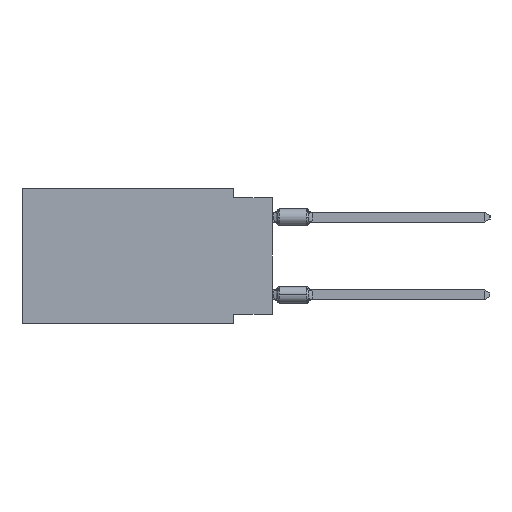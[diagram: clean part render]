
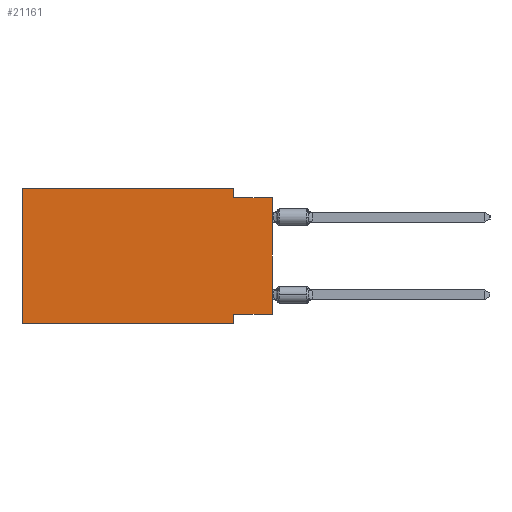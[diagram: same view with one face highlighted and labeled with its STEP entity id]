
A CAD part, left-side view. The second image highlights one B-rep face of the part: STEP entity #21161.
In plain terms, the highlighted planar face has unit normal (-1, 0, 0).
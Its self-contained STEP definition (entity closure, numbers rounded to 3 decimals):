
#135 = ORIENTED_EDGE ( 'NONE', *, *, #12241, .F. ) ;
#281 = EDGE_CURVE ( 'NONE', #18312, #9924, #28892, .T. ) ;
#1151 = CARTESIAN_POINT ( 'NONE',  ( 0., 0., -0.635 ) ) ;
#1558 = EDGE_CURVE ( 'NONE', #11872, #26297, #2142, .T. ) ;
#2047 = CARTESIAN_POINT ( 'NONE',  ( 0., 0., -8.255 ) ) ;
#2142 = LINE ( 'NONE', #33585, #17754 ) ;
#2963 = CARTESIAN_POINT ( 'NONE',  ( 0., 16.383, 0. ) ) ;
#4011 = CARTESIAN_POINT ( 'NONE',  ( 0., 16.383, -8.89 ) ) ;
#4338 = EDGE_CURVE ( 'NONE', #34104, #12734, #29491, .T. ) ;
#5373 = ORIENTED_EDGE ( 'NONE', *, *, #23506, .F. ) ;
#5751 = CARTESIAN_POINT ( 'NONE',  ( 0., 2.54, 0. ) ) ;
#7100 = EDGE_CURVE ( 'NONE', #11872, #12324, #21355, .T. ) ;
#7386 = VECTOR ( 'NONE', #18073, 1000. ) ;
#7520 = LINE ( 'NONE', #28800, #7386 ) ;
#7662 = EDGE_LOOP ( 'NONE', ( #23647, #9031, #10416, #135, #21304, #28058, #5373, #12961 ) ) ;
#8340 = DIRECTION ( 'NONE',  ( 1., 0., 0. ) ) ;
#8524 = DIRECTION ( 'NONE',  ( 0., 0., -1. ) ) ;
#8633 = EDGE_CURVE ( 'NONE', #18312, #16953, #19740, .T. ) ;
#9031 = ORIENTED_EDGE ( 'NONE', *, *, #22091, .F. ) ;
#9840 = DIRECTION ( 'NONE',  ( 0., 0., -1. ) ) ;
#9924 = VERTEX_POINT ( 'NONE', #2963 ) ;
#10416 = ORIENTED_EDGE ( 'NONE', *, *, #4338, .F. ) ;
#10452 = CARTESIAN_POINT ( 'NONE',  ( 0., 2.54, -8.89 ) ) ;
#10765 = FACE_OUTER_BOUND ( 'NONE', #7662, .T. ) ;
#11872 = VERTEX_POINT ( 'NONE', #2047 ) ;
#11925 = CARTESIAN_POINT ( 'NONE',  ( 0., 0., -0.635 ) ) ;
#12241 = EDGE_CURVE ( 'NONE', #9924, #34104, #7520, .T. ) ;
#12324 = VERTEX_POINT ( 'NONE', #13564 ) ;
#12609 = CARTESIAN_POINT ( 'NONE',  ( 0., 16.383, 0. ) ) ;
#12734 = VERTEX_POINT ( 'NONE', #18708 ) ;
#12784 = AXIS2_PLACEMENT_3D ( 'NONE', #31692, #8340, #8524 ) ;
#12961 = ORIENTED_EDGE ( 'NONE', *, *, #7100, .F. ) ;
#13564 = CARTESIAN_POINT ( 'NONE',  ( 0., 2.54, -8.255 ) ) ;
#16063 = VECTOR ( 'NONE', #9840, 1000. ) ;
#16627 = VECTOR ( 'NONE', #30184, 1000. ) ;
#16953 = VERTEX_POINT ( 'NONE', #10452 ) ;
#17480 = CARTESIAN_POINT ( 'NONE',  ( 0., 2.54, -8.89 ) ) ;
#17754 = VECTOR ( 'NONE', #28763, 1000. ) ;
#18073 = DIRECTION ( 'NONE',  ( 0., -1., 0. ) ) ;
#18312 = VERTEX_POINT ( 'NONE', #34023 ) ;
#18708 = CARTESIAN_POINT ( 'NONE',  ( 0., 2.54, -0.635 ) ) ;
#19740 = LINE ( 'NONE', #4011, #24284 ) ;
#21161 = ADVANCED_FACE ( 'NONE', ( #10765 ), #21316, .F. ) ;
#21304 = ORIENTED_EDGE ( 'NONE', *, *, #281, .F. ) ;
#21316 = PLANE ( 'NONE',  #12784 ) ;
#21355 = LINE ( 'NONE', #31887, #28816 ) ;
#22091 = EDGE_CURVE ( 'NONE', #12734, #26297, #28084, .T. ) ;
#22669 = VECTOR ( 'NONE', #23172, 1000. ) ;
#23172 = DIRECTION ( 'NONE',  ( 0., 0., 1. ) ) ;
#23506 = EDGE_CURVE ( 'NONE', #12324, #16953, #33042, .T. ) ;
#23647 = ORIENTED_EDGE ( 'NONE', *, *, #1558, .T. ) ;
#23767 = DIRECTION ( 'NONE',  ( 0., 1., 0. ) ) ;
#24264 = VECTOR ( 'NONE', #27061, 1000. ) ;
#24284 = VECTOR ( 'NONE', #25612, 1000. ) ;
#25612 = DIRECTION ( 'NONE',  ( 0., -1., 0. ) ) ;
#26297 = VERTEX_POINT ( 'NONE', #11925 ) ;
#27061 = DIRECTION ( 'NONE',  ( 0., 0., -1. ) ) ;
#28058 = ORIENTED_EDGE ( 'NONE', *, *, #8633, .T. ) ;
#28084 = LINE ( 'NONE', #1151, #16627 ) ;
#28763 = DIRECTION ( 'NONE',  ( 0., 0., 1. ) ) ;
#28800 = CARTESIAN_POINT ( 'NONE',  ( 0., 16.383, 0. ) ) ;
#28816 = VECTOR ( 'NONE', #23767, 1000. ) ;
#28892 = LINE ( 'NONE', #12609, #22669 ) ;
#29491 = LINE ( 'NONE', #29812, #24264 ) ;
#29812 = CARTESIAN_POINT ( 'NONE',  ( 0., 2.54, 0. ) ) ;
#30184 = DIRECTION ( 'NONE',  ( 0., -1., 0. ) ) ;
#31692 = CARTESIAN_POINT ( 'NONE',  ( 0., 16.383, 0. ) ) ;
#31887 = CARTESIAN_POINT ( 'NONE',  ( 0., 0., -8.255 ) ) ;
#33042 = LINE ( 'NONE', #17480, #16063 ) ;
#33585 = CARTESIAN_POINT ( 'NONE',  ( 0., 0., 0. ) ) ;
#34023 = CARTESIAN_POINT ( 'NONE',  ( 0., 16.383, -8.89 ) ) ;
#34104 = VERTEX_POINT ( 'NONE', #5751 ) ;
